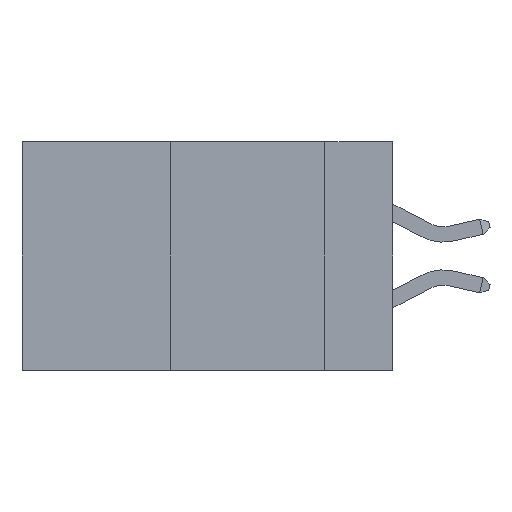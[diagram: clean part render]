
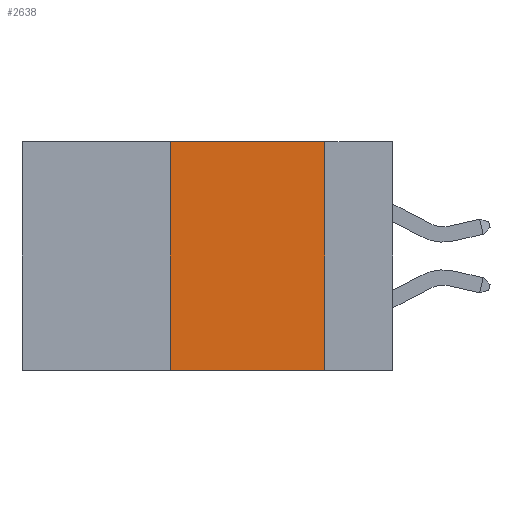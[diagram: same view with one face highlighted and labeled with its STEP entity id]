
A CAD part, left-side view. The second image highlights one B-rep face of the part: STEP entity #2638.
In plain terms, the highlighted planar face has unit normal (-1, 0, 0).
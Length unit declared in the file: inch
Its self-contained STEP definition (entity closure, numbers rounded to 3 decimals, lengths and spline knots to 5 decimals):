
#507 = VERTEX_POINT ( 'NONE', #29058 ) ;
#623 = EDGE_CURVE ( 'NONE', #19708, #507, #31299, .T. ) ;
#2638 = ADVANCED_FACE ( 'NONE', ( #33069 ), #10388, .F. ) ;
#3051 = ORIENTED_EDGE ( 'NONE', *, *, #32581, .F. ) ;
#3463 = CARTESIAN_POINT ( 'NONE',  ( 0., 0.36, -0.37 ) ) ;
#4295 = CARTESIAN_POINT ( 'NONE',  ( 0., 0.11, 0. ) ) ;
#5158 = LINE ( 'NONE', #4295, #20438 ) ;
#7285 = CARTESIAN_POINT ( 'NONE',  ( 0., 0.6, 0. ) ) ;
#7374 = DIRECTION ( 'NONE',  ( 0., 0., -1. ) ) ;
#7442 = LINE ( 'NONE', #37995, #38523 ) ;
#8886 = CARTESIAN_POINT ( 'NONE',  ( 0., 0.6, -0.37 ) ) ;
#10388 = PLANE ( 'NONE',  #12545 ) ;
#11100 = DIRECTION ( 'NONE',  ( 0., 0., 1. ) ) ;
#12012 = DIRECTION ( 'NONE',  ( 0., -1., 0. ) ) ;
#12545 = AXIS2_PLACEMENT_3D ( 'NONE', #7285, #19311, #13503 ) ;
#13503 = DIRECTION ( 'NONE',  ( 0., 0., -1. ) ) ;
#14545 = ORIENTED_EDGE ( 'NONE', *, *, #23580, .F. ) ;
#17806 = CARTESIAN_POINT ( 'NONE',  ( 0., 0.6, 0. ) ) ;
#19311 = DIRECTION ( 'NONE',  ( 1., 0., 0. ) ) ;
#19708 = VERTEX_POINT ( 'NONE', #29697 ) ;
#20438 = VECTOR ( 'NONE', #7374, 39.37008 ) ;
#20532 = EDGE_CURVE ( 'NONE', #24803, #21883, #28682, .T. ) ;
#21150 = ORIENTED_EDGE ( 'NONE', *, *, #20532, .T. ) ;
#21883 = VERTEX_POINT ( 'NONE', #35801 ) ;
#23580 = EDGE_CURVE ( 'NONE', #507, #21883, #5158, .T. ) ;
#24803 = VERTEX_POINT ( 'NONE', #3463 ) ;
#28682 = LINE ( 'NONE', #8886, #34734 ) ;
#29058 = CARTESIAN_POINT ( 'NONE',  ( 0., 0.11, 0. ) ) ;
#29697 = CARTESIAN_POINT ( 'NONE',  ( 0., 0.36, 0. ) ) ;
#30794 = EDGE_LOOP ( 'NONE', ( #14545, #32370, #3051, #21150 ) ) ;
#31299 = LINE ( 'NONE', #17806, #32220 ) ;
#32220 = VECTOR ( 'NONE', #38651, 39.37008 ) ;
#32370 = ORIENTED_EDGE ( 'NONE', *, *, #623, .F. ) ;
#32581 = EDGE_CURVE ( 'NONE', #24803, #19708, #7442, .T. ) ;
#33069 = FACE_OUTER_BOUND ( 'NONE', #30794, .T. ) ;
#34734 = VECTOR ( 'NONE', #12012, 39.37008 ) ;
#35801 = CARTESIAN_POINT ( 'NONE',  ( 0., 0.11, -0.37 ) ) ;
#37995 = CARTESIAN_POINT ( 'NONE',  ( 0., 0.36, 0. ) ) ;
#38523 = VECTOR ( 'NONE', #11100, 39.37008 ) ;
#38651 = DIRECTION ( 'NONE',  ( 0., -1., 0. ) ) ;
